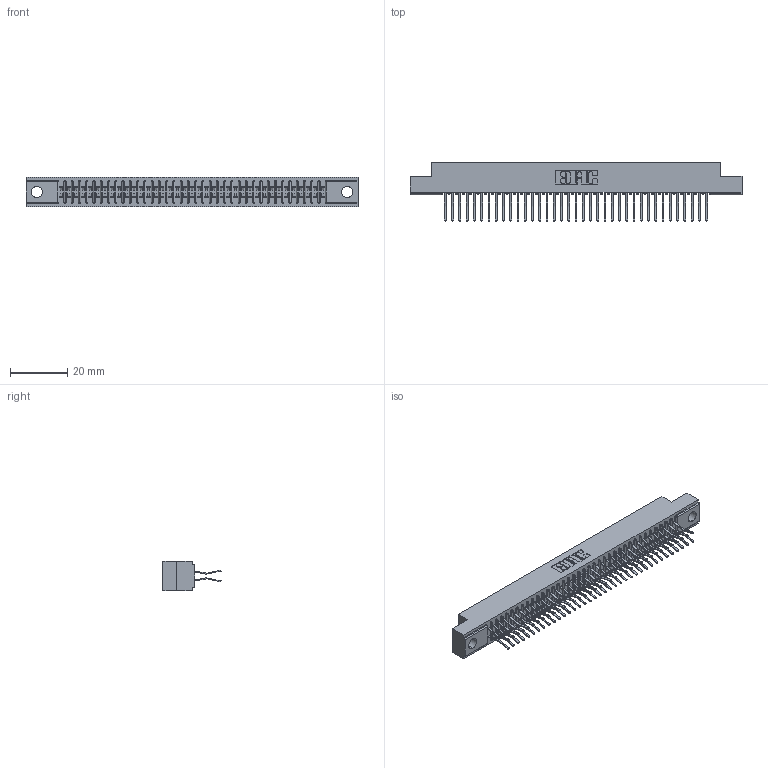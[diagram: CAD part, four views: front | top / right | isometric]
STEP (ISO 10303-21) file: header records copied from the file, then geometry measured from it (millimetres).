
FILE_DESCRIPTION (( 'STEP AP203' ), '1' );
FILE_NAME ('341-074-560-204.STEP', '2018-08-07T20:36:28', ( '' ), ( '' ), 'SwSTEP 2.0', 'SolidWorks 2016', '' );
FILE_SCHEMA (( 'CONFIG_CONTROL_DESIGN' ));
Length unit declared in the file: inch
Products named in the file (3): 341 Part_.156 (3.96) Dia Mounting Holes; 341-292-001_341-292-160; 341-074-560-204
Assembly tree (75 placements, depth 2):
  341-074-560-204
    341 Part_.156 (3.96) Dia Mounting Holes
    341-292-001_341-292-160  x74
Bounding box: 116.2 x 20.37 x 10.16 mm (x, y, z)
Volume: 8544.3 mm3; surface area: 15443.5 mm2
Topology: 75 solids, 75 shells, 5310 faces, 15411 edges, 9998 vertices
Faces by surface type: plane 3042, cylinder 2120, sphere 76, torus 72
Entity records: 46002 total; most frequent: CARTESIAN_POINT 7653, ORIENTED_EDGE 7602, DIRECTION 7427, EDGE_CURVE 3801, VECTOR 3067, LINE 3067, VERTEX_POINT 2406, AXIS2_PLACEMENT_3D 2180
